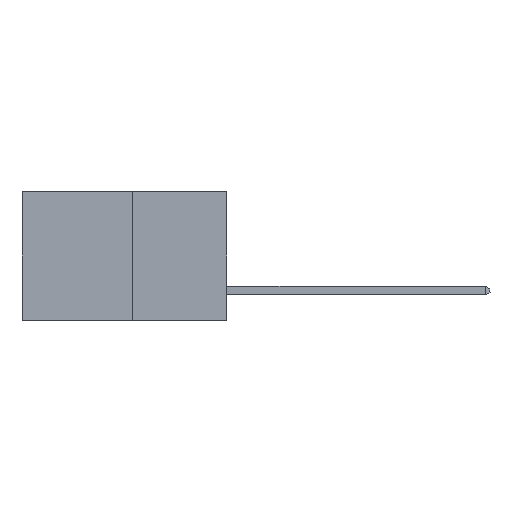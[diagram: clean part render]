
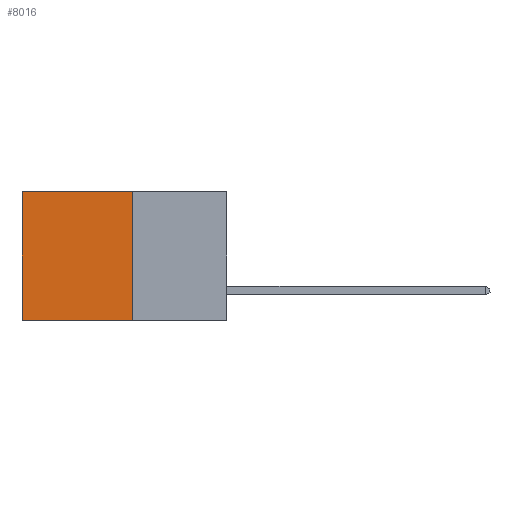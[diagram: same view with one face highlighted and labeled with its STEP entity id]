
A CAD part, left-side view. The second image highlights one B-rep face of the part: STEP entity #8016.
In plain terms, the highlighted planar face has unit normal (-1, 0, 0).
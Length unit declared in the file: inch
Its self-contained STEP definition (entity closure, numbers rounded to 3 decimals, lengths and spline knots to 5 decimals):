
#400 = VECTOR ( 'NONE', #7761, 39.37008 ) ;
#440 = ORIENTED_EDGE ( 'NONE', *, *, #5785, .T. ) ;
#1371 = CARTESIAN_POINT ( 'NONE',  ( 0.277, 0.59, -0.37 ) ) ;
#1548 = CARTESIAN_POINT ( 'NONE',  ( 0.277, 0.27, -0.37 ) ) ;
#1657 = LINE ( 'NONE', #6835, #8542 ) ;
#2302 = VECTOR ( 'NONE', #4997, 39.37008 ) ;
#2521 = VERTEX_POINT ( 'NONE', #5030 ) ;
#3317 = VERTEX_POINT ( 'NONE', #8830 ) ;
#3633 = EDGE_CURVE ( 'NONE', #2521, #6673, #1657, .T. ) ;
#3860 = VECTOR ( 'NONE', #6964, 39.37008 ) ;
#3968 = ORIENTED_EDGE ( 'NONE', *, *, #8203, .F. ) ;
#4121 = DIRECTION ( 'NONE',  ( 0., 0., -1. ) ) ;
#4867 = AXIS2_PLACEMENT_3D ( 'NONE', #7574, #8213, #4121 ) ;
#4997 = DIRECTION ( 'NONE',  ( 0., 0., -1. ) ) ;
#5030 = CARTESIAN_POINT ( 'NONE',  ( 0.277, 0.27, -0.37 ) ) ;
#5455 = PLANE ( 'NONE',  #4867 ) ;
#5473 = EDGE_LOOP ( 'NONE', ( #7224, #5581, #3968, #440 ) ) ;
#5581 = ORIENTED_EDGE ( 'NONE', *, *, #3633, .F. ) ;
#5785 = EDGE_CURVE ( 'NONE', #7845, #3317, #7813, .T. ) ;
#5932 = CARTESIAN_POINT ( 'NONE',  ( 0.277, 0.27, 0. ) ) ;
#6135 = FACE_OUTER_BOUND ( 'NONE', #5473, .T. ) ;
#6633 = CARTESIAN_POINT ( 'NONE',  ( 0.277, 0.59, -0.37 ) ) ;
#6673 = VERTEX_POINT ( 'NONE', #6633 ) ;
#6835 = CARTESIAN_POINT ( 'NONE',  ( 0.277, 0.27, -0.37 ) ) ;
#6964 = DIRECTION ( 'NONE',  ( 0., 0., -1. ) ) ;
#7040 = CARTESIAN_POINT ( 'NONE',  ( 0.277, 0.27, 0. ) ) ;
#7224 = ORIENTED_EDGE ( 'NONE', *, *, #8052, .T. ) ;
#7321 = LINE ( 'NONE', #1371, #3860 ) ;
#7574 = CARTESIAN_POINT ( 'NONE',  ( 0.277, 0.27, -0.37 ) ) ;
#7761 = DIRECTION ( 'NONE',  ( 0., 1., 0. ) ) ;
#7813 = LINE ( 'NONE', #7040, #400 ) ;
#7832 = LINE ( 'NONE', #1548, #2302 ) ;
#7845 = VERTEX_POINT ( 'NONE', #5932 ) ;
#8016 = ADVANCED_FACE ( 'NONE', ( #6135 ), #5455, .F. ) ;
#8052 = EDGE_CURVE ( 'NONE', #3317, #6673, #7321, .T. ) ;
#8203 = EDGE_CURVE ( 'NONE', #7845, #2521, #7832, .T. ) ;
#8213 = DIRECTION ( 'NONE',  ( 1., 0., 0. ) ) ;
#8542 = VECTOR ( 'NONE', #8858, 39.37008 ) ;
#8830 = CARTESIAN_POINT ( 'NONE',  ( 0.277, 0.59, 0. ) ) ;
#8858 = DIRECTION ( 'NONE',  ( 0., 1., 0. ) ) ;
